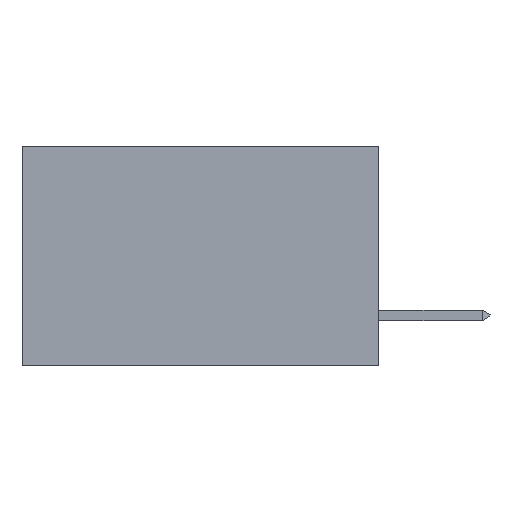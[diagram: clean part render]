
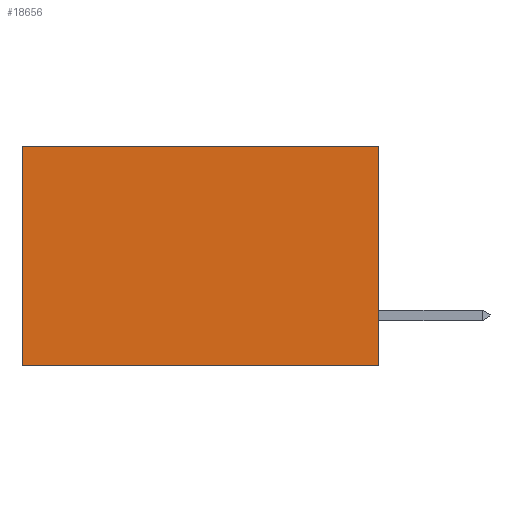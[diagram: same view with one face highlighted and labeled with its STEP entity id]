
A CAD part, left-side view. The second image highlights one B-rep face of the part: STEP entity #18656.
In plain terms, the highlighted planar face has unit normal (-1, 0, 0).
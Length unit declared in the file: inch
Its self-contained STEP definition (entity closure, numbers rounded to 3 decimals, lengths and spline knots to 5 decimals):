
#236 = CARTESIAN_POINT ( 'NONE',  ( 0.298, 0., 0. ) ) ;
#246 = ORIENTED_EDGE ( 'NONE', *, *, #9671, .T. ) ;
#365 = DIRECTION ( 'NONE',  ( 0., 1., 0. ) ) ;
#1444 = DIRECTION ( 'NONE',  ( 0., 0., -1. ) ) ;
#1522 = CARTESIAN_POINT ( 'NONE',  ( 0.298, 0., 0. ) ) ;
#1910 = VERTEX_POINT ( 'NONE', #5898 ) ;
#2358 = FACE_OUTER_BOUND ( 'NONE', #6601, .T. ) ;
#3490 = ORIENTED_EDGE ( 'NONE', *, *, #12584, .T. ) ;
#3917 = CARTESIAN_POINT ( 'NONE',  ( 0.298, 0.6, 0. ) ) ;
#5809 = EDGE_CURVE ( 'NONE', #19049, #16386, #12579, .T. ) ;
#5898 = CARTESIAN_POINT ( 'NONE',  ( 0.298, 0.6, -0.37 ) ) ;
#6601 = EDGE_LOOP ( 'NONE', ( #3490, #12361, #20785, #246 ) ) ;
#8860 = LINE ( 'NONE', #19312, #11716 ) ;
#9671 = EDGE_CURVE ( 'NONE', #19049, #21404, #20144, .T. ) ;
#9926 = EDGE_CURVE ( 'NONE', #16386, #1910, #19272, .T. ) ;
#11268 = CARTESIAN_POINT ( 'NONE',  ( 0.298, 0., -0.37 ) ) ;
#11569 = PLANE ( 'NONE',  #18664 ) ;
#11716 = VECTOR ( 'NONE', #12000, 39.37008 ) ;
#12000 = DIRECTION ( 'NONE',  ( 0., 0., -1. ) ) ;
#12361 = ORIENTED_EDGE ( 'NONE', *, *, #9926, .F. ) ;
#12579 = LINE ( 'NONE', #1522, #19195 ) ;
#12584 = EDGE_CURVE ( 'NONE', #21404, #1910, #8860, .T. ) ;
#12977 = CARTESIAN_POINT ( 'NONE',  ( 0.298, 0., 0. ) ) ;
#14381 = VECTOR ( 'NONE', #365, 39.37008 ) ;
#15257 = VECTOR ( 'NONE', #17037, 39.37008 ) ;
#15555 = DIRECTION ( 'NONE',  ( 1., 0., 0. ) ) ;
#16386 = VERTEX_POINT ( 'NONE', #23653 ) ;
#17037 = DIRECTION ( 'NONE',  ( 0., 1., 0. ) ) ;
#18656 = ADVANCED_FACE ( 'NONE', ( #2358 ), #11569, .F. ) ;
#18664 = AXIS2_PLACEMENT_3D ( 'NONE', #21011, #15555, #21088 ) ;
#19049 = VERTEX_POINT ( 'NONE', #236 ) ;
#19195 = VECTOR ( 'NONE', #1444, 39.37008 ) ;
#19272 = LINE ( 'NONE', #11268, #14381 ) ;
#19312 = CARTESIAN_POINT ( 'NONE',  ( 0.298, 0.6, 0. ) ) ;
#20144 = LINE ( 'NONE', #12977, #15257 ) ;
#20785 = ORIENTED_EDGE ( 'NONE', *, *, #5809, .F. ) ;
#21011 = CARTESIAN_POINT ( 'NONE',  ( 0.298, 0., 0. ) ) ;
#21088 = DIRECTION ( 'NONE',  ( 0., 0., -1. ) ) ;
#21404 = VERTEX_POINT ( 'NONE', #3917 ) ;
#23653 = CARTESIAN_POINT ( 'NONE',  ( 0.298, 0., -0.37 ) ) ;
